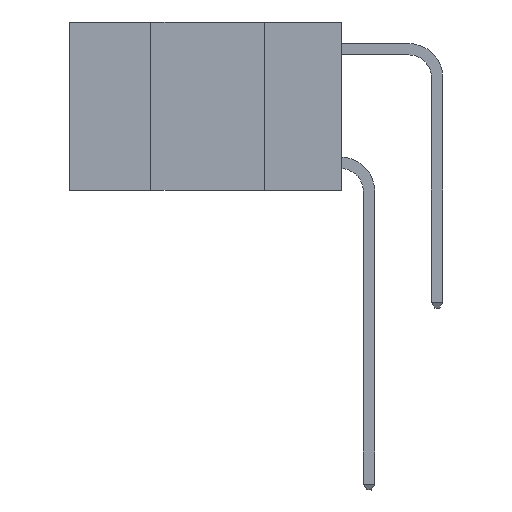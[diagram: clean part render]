
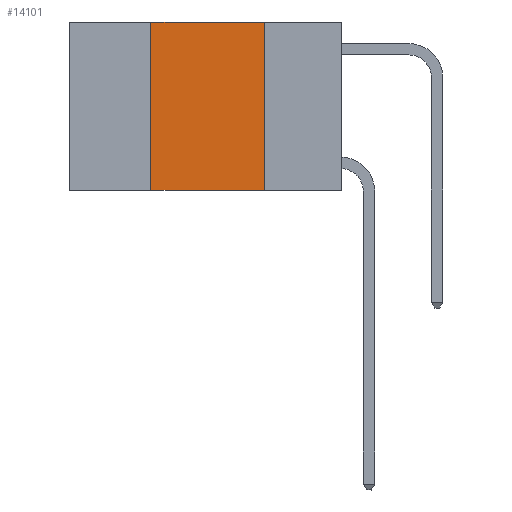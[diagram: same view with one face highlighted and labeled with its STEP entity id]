
A CAD part, left-side view. The second image highlights one B-rep face of the part: STEP entity #14101.
In plain terms, the highlighted planar face has unit normal (-1, 0, 0).
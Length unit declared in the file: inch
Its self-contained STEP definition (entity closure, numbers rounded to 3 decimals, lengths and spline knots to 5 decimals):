
#962 = EDGE_CURVE ( 'NONE', #12267, #3468, #18808, .T. ) ;
#1737 = DIRECTION ( 'NONE',  ( 0., -1., 0. ) ) ;
#2168 = ORIENTED_EDGE ( 'NONE', *, *, #962, .F. ) ;
#2547 = VECTOR ( 'NONE', #1737, 39.37008 ) ;
#3224 = VERTEX_POINT ( 'NONE', #13190 ) ;
#3411 = AXIS2_PLACEMENT_3D ( 'NONE', #11390, #14517, #6758 ) ;
#3468 = VERTEX_POINT ( 'NONE', #15031 ) ;
#5240 = ORIENTED_EDGE ( 'NONE', *, *, #17991, .F. ) ;
#5775 = CARTESIAN_POINT ( 'NONE',  ( 0., 0.42, 0. ) ) ;
#6139 = VERTEX_POINT ( 'NONE', #5775 ) ;
#6236 = ORIENTED_EDGE ( 'NONE', *, *, #15208, .T. ) ;
#6758 = DIRECTION ( 'NONE',  ( 0., 0., -1. ) ) ;
#6927 = VECTOR ( 'NONE', #19058, 39.37008 ) ;
#7676 = CARTESIAN_POINT ( 'NONE',  ( 0., 0.42, 0. ) ) ;
#7712 = DIRECTION ( 'NONE',  ( 0., 0., -1. ) ) ;
#8852 = LINE ( 'NONE', #17054, #2547 ) ;
#9400 = FACE_OUTER_BOUND ( 'NONE', #15108, .T. ) ;
#9518 = CARTESIAN_POINT ( 'NONE',  ( 0., 0.6, 0. ) ) ;
#9671 = EDGE_CURVE ( 'NONE', #3224, #6139, #17028, .T. ) ;
#9987 = LINE ( 'NONE', #9518, #6927 ) ;
#10099 = VECTOR ( 'NONE', #7712, 39.37008 ) ;
#11390 = CARTESIAN_POINT ( 'NONE',  ( 0., 0.6, 0. ) ) ;
#11584 = PLANE ( 'NONE',  #3411 ) ;
#12267 = VERTEX_POINT ( 'NONE', #13488 ) ;
#13190 = CARTESIAN_POINT ( 'NONE',  ( 0., 0.42, -0.37 ) ) ;
#13488 = CARTESIAN_POINT ( 'NONE',  ( 0., 0.17, 0. ) ) ;
#13995 = DIRECTION ( 'NONE',  ( 0., 0., 1. ) ) ;
#14101 = ADVANCED_FACE ( 'NONE', ( #9400 ), #11584, .F. ) ;
#14517 = DIRECTION ( 'NONE',  ( 1., 0., 0. ) ) ;
#14592 = VECTOR ( 'NONE', #13995, 39.37008 ) ;
#15031 = CARTESIAN_POINT ( 'NONE',  ( 0., 0.17, -0.37 ) ) ;
#15108 = EDGE_LOOP ( 'NONE', ( #2168, #5240, #18878, #6236 ) ) ;
#15208 = EDGE_CURVE ( 'NONE', #3224, #3468, #8852, .T. ) ;
#17028 = LINE ( 'NONE', #7676, #14592 ) ;
#17054 = CARTESIAN_POINT ( 'NONE',  ( 0., 0.6, -0.37 ) ) ;
#17991 = EDGE_CURVE ( 'NONE', #6139, #12267, #9987, .T. ) ;
#18022 = CARTESIAN_POINT ( 'NONE',  ( 0., 0.17, 0. ) ) ;
#18808 = LINE ( 'NONE', #18022, #10099 ) ;
#18878 = ORIENTED_EDGE ( 'NONE', *, *, #9671, .F. ) ;
#19058 = DIRECTION ( 'NONE',  ( 0., -1., 0. ) ) ;
